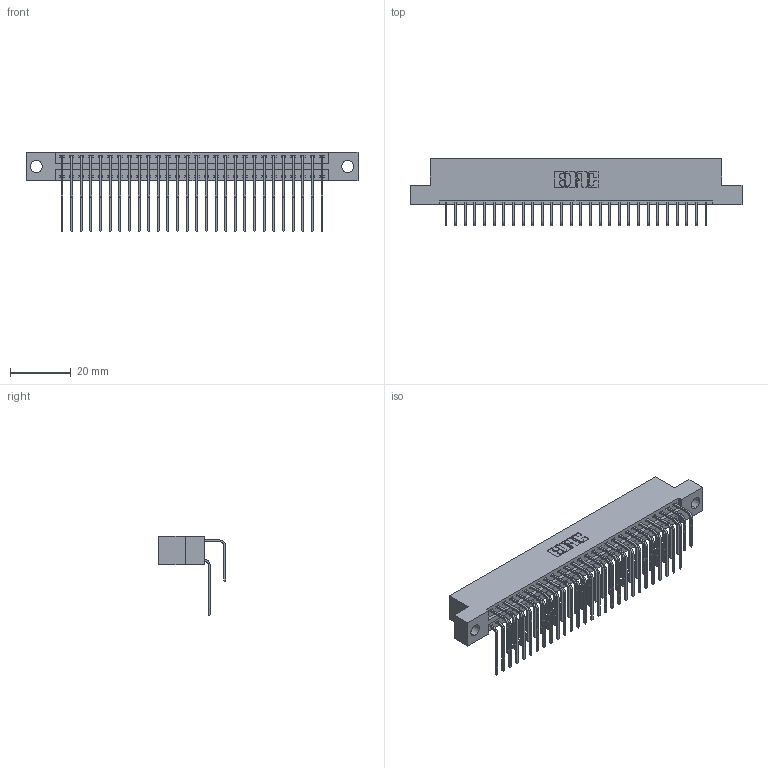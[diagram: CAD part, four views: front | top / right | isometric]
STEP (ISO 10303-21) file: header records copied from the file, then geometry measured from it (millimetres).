
FILE_DESCRIPTION (( 'STEP AP203' ), '1' );
FILE_NAME ('346-056-558-204.STEP', '2022-05-21T06:40:16', ( '' ), ( '' ), 'SwSTEP 2.0', 'SolidWorks 2020', '' );
FILE_SCHEMA (( 'CONFIG_CONTROL_DESIGN' ));
Length unit declared in the file: inch
Products named in the file (4): 345-292-001_558 Tail - 2; 346 Part_Flush Mounting Lugs - 0.156 Dia-TH; 346-056-558-204; 345-292-001_558 559 Tail - 1
Assembly tree (57 placements, depth 2):
  346-056-558-204
    346 Part_Flush Mounting Lugs - 0.156 Dia-TH
    345-292-001_558 559 Tail - 1  x28
    345-292-001_558 Tail - 2  x28
Bounding box: 109.47 x 22.16 x 26.16 mm (x, y, z)
Volume: 10783.4 mm3; surface area: 16000.2 mm2
Topology: 57 solids, 57 shells, 3160 faces, 9381 edges, 6178 vertices
Faces by surface type: plane 2162, cylinder 998
Entity records: 22361 total; most frequent: CARTESIAN_POINT 3761, ORIENTED_EDGE 3642, DIRECTION 3337, EDGE_CURVE 1821, VECTOR 1537, LINE 1537, VERTEX_POINT 1210, AXIS2_PLACEMENT_3D 900
